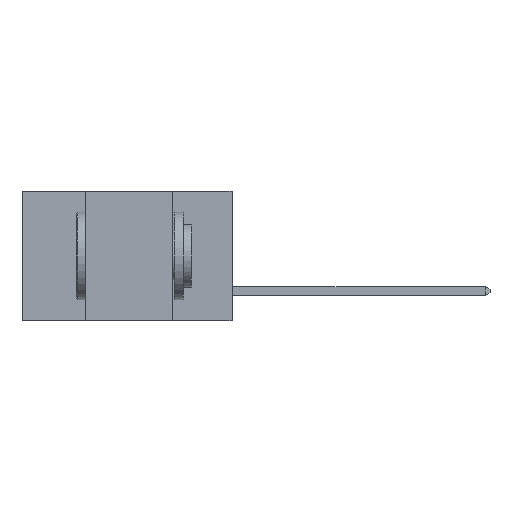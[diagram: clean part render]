
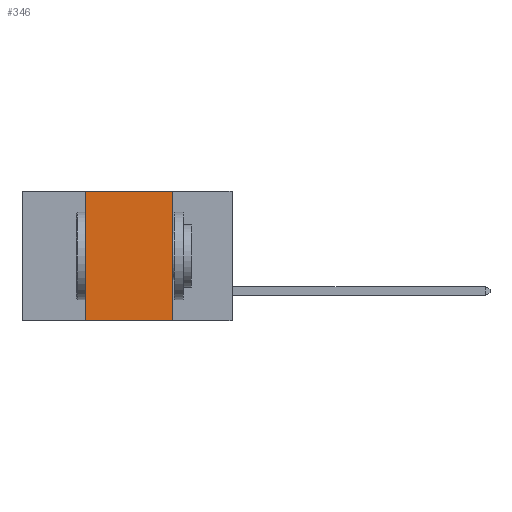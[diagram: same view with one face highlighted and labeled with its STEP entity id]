
A CAD part, left-side view. The second image highlights one B-rep face of the part: STEP entity #346.
In plain terms, the highlighted planar face has unit normal (-1, 0, 0).
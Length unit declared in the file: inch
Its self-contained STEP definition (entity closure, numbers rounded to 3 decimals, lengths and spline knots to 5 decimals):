
#273 = ORIENTED_EDGE ( 'NONE', *, *, #792, .F. ) ;
#346 = ADVANCED_FACE ( 'NONE', ( #2076 ), #4017, .F. ) ;
#792 = EDGE_CURVE ( 'NONE', #5473, #7037, #4277, .T. ) ;
#951 = EDGE_CURVE ( 'NONE', #7037, #3906, #4842, .T. ) ;
#953 = ORIENTED_EDGE ( 'NONE', *, *, #951, .F. ) ;
#1296 = DIRECTION ( 'NONE',  ( 0., -1., 0. ) ) ;
#1418 = CARTESIAN_POINT ( 'NONE',  ( 0., 0.17, 0. ) ) ;
#1576 = DIRECTION ( 'NONE',  ( 1., 0., 0. ) ) ;
#1821 = ORIENTED_EDGE ( 'NONE', *, *, #2866, .F. ) ;
#2076 = FACE_OUTER_BOUND ( 'NONE', #2475, .T. ) ;
#2375 = CARTESIAN_POINT ( 'NONE',  ( 0., 0.17, -0.37 ) ) ;
#2475 = EDGE_LOOP ( 'NONE', ( #1821, #953, #273, #4207 ) ) ;
#2635 = DIRECTION ( 'NONE',  ( 0., 0., -1. ) ) ;
#2648 = CARTESIAN_POINT ( 'NONE',  ( 0., 0.6, 0. ) ) ;
#2656 = DIRECTION ( 'NONE',  ( 0., -1., 0. ) ) ;
#2866 = EDGE_CURVE ( 'NONE', #3906, #3817, #3363, .T. ) ;
#2874 = CARTESIAN_POINT ( 'NONE',  ( 0., 0.6, -0.37 ) ) ;
#3184 = DIRECTION ( 'NONE',  ( 0., 0., 1. ) ) ;
#3363 = LINE ( 'NONE', #9064, #8752 ) ;
#3404 = AXIS2_PLACEMENT_3D ( 'NONE', #9148, #1576, #2635 ) ;
#3738 = CARTESIAN_POINT ( 'NONE',  ( 0., 0.42, 0. ) ) ;
#3817 = VERTEX_POINT ( 'NONE', #2375 ) ;
#3906 = VERTEX_POINT ( 'NONE', #1418 ) ;
#4017 = PLANE ( 'NONE',  #3404 ) ;
#4207 = ORIENTED_EDGE ( 'NONE', *, *, #8278, .T. ) ;
#4277 = LINE ( 'NONE', #3738, #6192 ) ;
#4842 = LINE ( 'NONE', #2648, #8270 ) ;
#5006 = LINE ( 'NONE', #2874, #8422 ) ;
#5473 = VERTEX_POINT ( 'NONE', #7709 ) ;
#6192 = VECTOR ( 'NONE', #3184, 39.37008 ) ;
#7037 = VERTEX_POINT ( 'NONE', #8608 ) ;
#7709 = CARTESIAN_POINT ( 'NONE',  ( 0., 0.42, -0.37 ) ) ;
#8270 = VECTOR ( 'NONE', #2656, 39.37008 ) ;
#8278 = EDGE_CURVE ( 'NONE', #5473, #3817, #5006, .T. ) ;
#8422 = VECTOR ( 'NONE', #1296, 39.37008 ) ;
#8608 = CARTESIAN_POINT ( 'NONE',  ( 0., 0.42, 0. ) ) ;
#8752 = VECTOR ( 'NONE', #8925, 39.37008 ) ;
#8925 = DIRECTION ( 'NONE',  ( 0., 0., -1. ) ) ;
#9064 = CARTESIAN_POINT ( 'NONE',  ( 0., 0.17, 0. ) ) ;
#9148 = CARTESIAN_POINT ( 'NONE',  ( 0., 0.6, 0. ) ) ;
